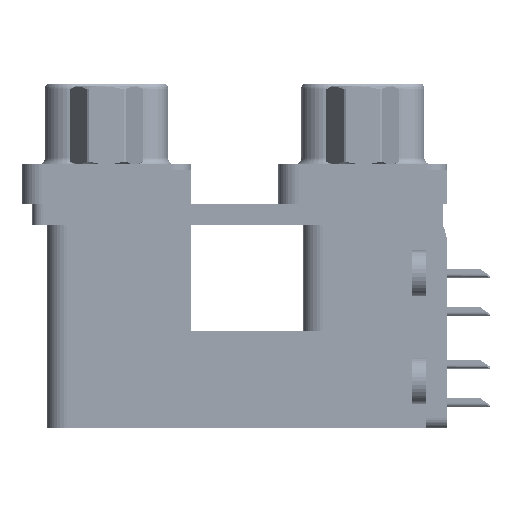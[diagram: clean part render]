
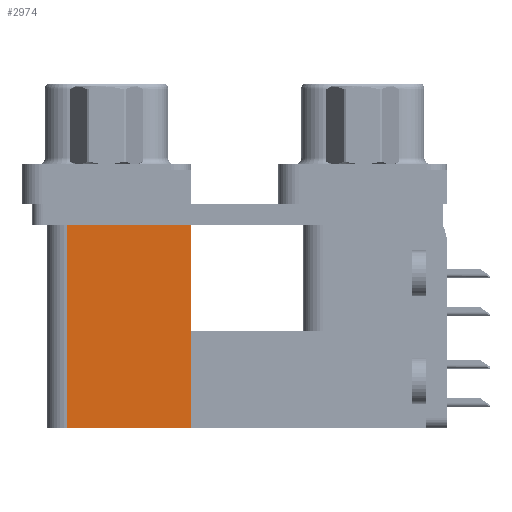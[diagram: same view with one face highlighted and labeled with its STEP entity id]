
A CAD part, left-side view. The second image highlights one B-rep face of the part: STEP entity #2974.
In plain terms, the highlighted planar face has unit normal (-1, 0, 0).
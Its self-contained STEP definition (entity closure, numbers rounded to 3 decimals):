
#2974 = ADVANCED_FACE ( 'NONE', ( #34012 ), #6676, .F. ) ;
#3828 = EDGE_CURVE ( 'NONE', #5435, #13289, #24758, .T. ) ;
#4341 = DIRECTION ( 'NONE',  ( 0., 0., 1. ) ) ;
#5435 = VERTEX_POINT ( 'NONE', #18776 ) ;
#6676 = PLANE ( 'NONE',  #12253 ) ;
#8473 = CARTESIAN_POINT ( 'NONE',  ( 3.79, 12.775, -19.2 ) ) ;
#8556 = VERTEX_POINT ( 'NONE', #37598 ) ;
#10417 = ORIENTED_EDGE ( 'NONE', *, *, #14385, .F. ) ;
#12253 = AXIS2_PLACEMENT_3D ( 'NONE', #41964, #55765, #28739 ) ;
#13289 = VERTEX_POINT ( 'NONE', #53468 ) ;
#14385 = EDGE_CURVE ( 'NONE', #13289, #8556, #18334, .T. ) ;
#15330 = VECTOR ( 'NONE', #27425, 1000. ) ;
#15640 = CARTESIAN_POINT ( 'NONE',  ( 3.79, 12.775, -19.2 ) ) ;
#17977 = LINE ( 'NONE', #48006, #31627 ) ;
#18334 = LINE ( 'NONE', #48925, #15330 ) ;
#18776 = CARTESIAN_POINT ( 'NONE',  ( 3.79, 12.775, -19.2 ) ) ;
#19754 = DIRECTION ( 'NONE',  ( 0., 1., 0. ) ) ;
#19958 = EDGE_CURVE ( 'NONE', #39883, #8556, #17977, .T. ) ;
#24291 = ORIENTED_EDGE ( 'NONE', *, *, #19958, .T. ) ;
#24758 = LINE ( 'NONE', #15640, #30274 ) ;
#27425 = DIRECTION ( 'NONE',  ( 0., 0., 1. ) ) ;
#27513 = EDGE_LOOP ( 'NONE', ( #24291, #10417, #55984, #36599 ) ) ;
#28739 = DIRECTION ( 'NONE',  ( 0., 0., -1. ) ) ;
#30274 = VECTOR ( 'NONE', #19754, 1000. ) ;
#31627 = VECTOR ( 'NONE', #35910, 1000. ) ;
#31809 = VECTOR ( 'NONE', #4341, 1000. ) ;
#34012 = FACE_OUTER_BOUND ( 'NONE', #27513, .T. ) ;
#34643 = EDGE_CURVE ( 'NONE', #5435, #39883, #48740, .T. ) ;
#35910 = DIRECTION ( 'NONE',  ( 0., 1., 0. ) ) ;
#36599 = ORIENTED_EDGE ( 'NONE', *, *, #34643, .T. ) ;
#37598 = CARTESIAN_POINT ( 'NONE',  ( 3.79, 21.975, -2.5 ) ) ;
#39883 = VERTEX_POINT ( 'NONE', #50861 ) ;
#41964 = CARTESIAN_POINT ( 'NONE',  ( 3.79, 12.775, -19.2 ) ) ;
#48006 = CARTESIAN_POINT ( 'NONE',  ( 3.79, 12.775, -2.5 ) ) ;
#48740 = LINE ( 'NONE', #8473, #31809 ) ;
#48925 = CARTESIAN_POINT ( 'NONE',  ( 3.79, 21.975, -19.2 ) ) ;
#50861 = CARTESIAN_POINT ( 'NONE',  ( 3.79, 12.775, -2.5 ) ) ;
#53468 = CARTESIAN_POINT ( 'NONE',  ( 3.79, 21.975, -19.2 ) ) ;
#55765 = DIRECTION ( 'NONE',  ( 1., 0., 0. ) ) ;
#55984 = ORIENTED_EDGE ( 'NONE', *, *, #3828, .F. ) ;
